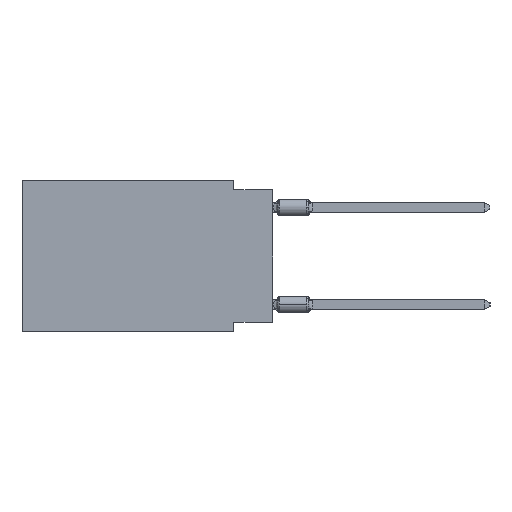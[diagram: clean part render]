
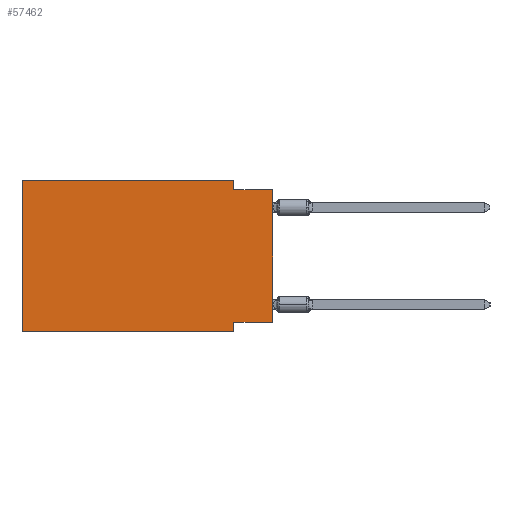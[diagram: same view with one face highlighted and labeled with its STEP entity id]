
A CAD part, left-side view. The second image highlights one B-rep face of the part: STEP entity #57462.
In plain terms, the highlighted planar face has unit normal (-1, 0, 0).
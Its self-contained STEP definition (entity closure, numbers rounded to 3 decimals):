
#348 = ORIENTED_EDGE ( 'NONE', *, *, #21371, .T. ) ;
#577 = DIRECTION ( 'NONE',  ( 0., -1., 0. ) ) ;
#1014 = ORIENTED_EDGE ( 'NONE', *, *, #9391, .T. ) ;
#1311 = VECTOR ( 'NONE', #9615, 1000. ) ;
#1439 = LINE ( 'NONE', #34086, #57135 ) ;
#3322 = VERTEX_POINT ( 'NONE', #32248 ) ;
#3488 = CARTESIAN_POINT ( 'NONE',  ( 0., 2.54, -9.906 ) ) ;
#3717 = DIRECTION ( 'NONE',  ( 0., 0., 1. ) ) ;
#5117 = CARTESIAN_POINT ( 'NONE',  ( 0., 16.383, -9.906 ) ) ;
#7845 = CARTESIAN_POINT ( 'NONE',  ( 0., 2.54, 0. ) ) ;
#8101 = CARTESIAN_POINT ( 'NONE',  ( 0., 16.383, -9.906 ) ) ;
#8844 = VECTOR ( 'NONE', #3717, 1000. ) ;
#9144 = VERTEX_POINT ( 'NONE', #7845 ) ;
#9391 = EDGE_CURVE ( 'NONE', #24683, #31623, #50633, .T. ) ;
#9615 = DIRECTION ( 'NONE',  ( 0., -1., 0. ) ) ;
#10041 = ORIENTED_EDGE ( 'NONE', *, *, #12262, .F. ) ;
#12083 = VERTEX_POINT ( 'NONE', #41616 ) ;
#12262 = EDGE_CURVE ( 'NONE', #3322, #39775, #1439, .T. ) ;
#12390 = EDGE_LOOP ( 'NONE', ( #348, #10041, #13658, #51319, #57913, #1014, #19033, #38089 ) ) ;
#12825 = FACE_OUTER_BOUND ( 'NONE', #12390, .T. ) ;
#13658 = ORIENTED_EDGE ( 'NONE', *, *, #56492, .F. ) ;
#14093 = LINE ( 'NONE', #23967, #57032 ) ;
#16541 = DIRECTION ( 'NONE',  ( 0., 0., -1. ) ) ;
#17002 = DIRECTION ( 'NONE',  ( 0., 0., -1. ) ) ;
#17565 = VERTEX_POINT ( 'NONE', #38595 ) ;
#19033 = ORIENTED_EDGE ( 'NONE', *, *, #22888, .F. ) ;
#19355 = CARTESIAN_POINT ( 'NONE',  ( 0., 16.383, 0. ) ) ;
#21371 = EDGE_CURVE ( 'NONE', #35868, #39775, #58223, .T. ) ;
#22888 = EDGE_CURVE ( 'NONE', #17565, #31623, #33917, .T. ) ;
#23967 = CARTESIAN_POINT ( 'NONE',  ( 0., 16.383, 0. ) ) ;
#24140 = CARTESIAN_POINT ( 'NONE',  ( 0., 2.54, 0. ) ) ;
#24683 = VERTEX_POINT ( 'NONE', #8101 ) ;
#25135 = VECTOR ( 'NONE', #42710, 1000. ) ;
#29568 = CARTESIAN_POINT ( 'NONE',  ( 0., 0., -9.271 ) ) ;
#31623 = VERTEX_POINT ( 'NONE', #3488 ) ;
#32248 = CARTESIAN_POINT ( 'NONE',  ( 0., 2.54, -0.635 ) ) ;
#33917 = LINE ( 'NONE', #47994, #52427 ) ;
#33987 = EDGE_CURVE ( 'NONE', #12083, #9144, #14093, .T. ) ;
#34086 = CARTESIAN_POINT ( 'NONE',  ( 0., 0., -0.635 ) ) ;
#35418 = VECTOR ( 'NONE', #39008, 1000. ) ;
#35792 = EDGE_CURVE ( 'NONE', #35868, #17565, #38543, .T. ) ;
#35868 = VERTEX_POINT ( 'NONE', #29568 ) ;
#37321 = LINE ( 'NONE', #19355, #25135 ) ;
#38089 = ORIENTED_EDGE ( 'NONE', *, *, #35792, .F. ) ;
#38543 = LINE ( 'NONE', #39143, #45272 ) ;
#38595 = CARTESIAN_POINT ( 'NONE',  ( 0., 2.54, -9.271 ) ) ;
#38840 = DIRECTION ( 'NONE',  ( 0., 1., 0. ) ) ;
#39008 = DIRECTION ( 'NONE',  ( 0., 0., -1. ) ) ;
#39143 = CARTESIAN_POINT ( 'NONE',  ( 0., 0., -9.271 ) ) ;
#39465 = PLANE ( 'NONE',  #47107 ) ;
#39775 = VERTEX_POINT ( 'NONE', #48057 ) ;
#41616 = CARTESIAN_POINT ( 'NONE',  ( 0., 16.383, 0. ) ) ;
#42710 = DIRECTION ( 'NONE',  ( 0., 0., 1. ) ) ;
#44764 = CARTESIAN_POINT ( 'NONE',  ( 0., 0., 0. ) ) ;
#45272 = VECTOR ( 'NONE', #38840, 1000. ) ;
#46601 = LINE ( 'NONE', #24140, #35418 ) ;
#47107 = AXIS2_PLACEMENT_3D ( 'NONE', #48437, #52914, #17002 ) ;
#47576 = DIRECTION ( 'NONE',  ( 0., -1., 0. ) ) ;
#47994 = CARTESIAN_POINT ( 'NONE',  ( 0., 2.54, -9.906 ) ) ;
#48057 = CARTESIAN_POINT ( 'NONE',  ( 0., 0., -0.635 ) ) ;
#48437 = CARTESIAN_POINT ( 'NONE',  ( 0., 16.383, 0. ) ) ;
#50633 = LINE ( 'NONE', #5117, #1311 ) ;
#51319 = ORIENTED_EDGE ( 'NONE', *, *, #33987, .F. ) ;
#52427 = VECTOR ( 'NONE', #16541, 1000. ) ;
#52914 = DIRECTION ( 'NONE',  ( 1., 0., 0. ) ) ;
#56492 = EDGE_CURVE ( 'NONE', #9144, #3322, #46601, .T. ) ;
#57032 = VECTOR ( 'NONE', #577, 1000. ) ;
#57135 = VECTOR ( 'NONE', #47576, 1000. ) ;
#57462 = ADVANCED_FACE ( 'NONE', ( #12825 ), #39465, .F. ) ;
#57769 = EDGE_CURVE ( 'NONE', #24683, #12083, #37321, .T. ) ;
#57913 = ORIENTED_EDGE ( 'NONE', *, *, #57769, .F. ) ;
#58223 = LINE ( 'NONE', #44764, #8844 ) ;
